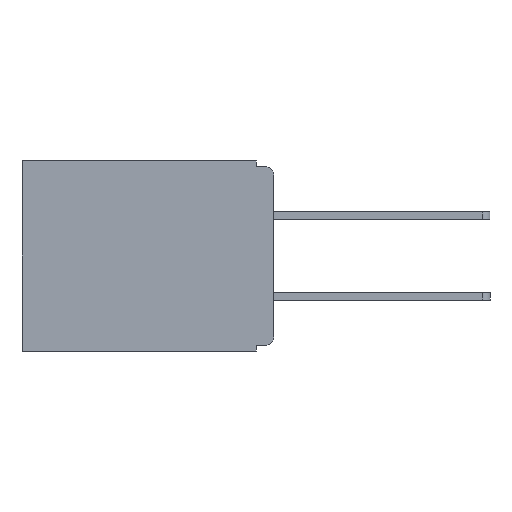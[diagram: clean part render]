
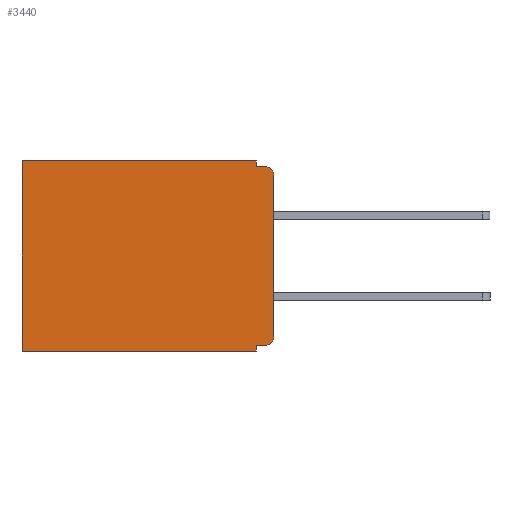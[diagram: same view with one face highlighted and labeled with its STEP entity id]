
A CAD part, left-side view. The second image highlights one B-rep face of the part: STEP entity #3440.
In plain terms, the highlighted planar face has unit normal (-1, 0, 0).
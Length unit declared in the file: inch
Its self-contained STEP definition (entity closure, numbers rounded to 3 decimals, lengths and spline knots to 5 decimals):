
#128 = EDGE_CURVE ( 'NONE', #9035, #3549, #1771, .T. ) ;
#164 = VERTEX_POINT ( 'NONE', #965 ) ;
#360 = EDGE_CURVE ( 'NONE', #1878, #3993, #12144, .T. ) ;
#444 = AXIS2_PLACEMENT_3D ( 'NONE', #8846, #1423, #1316 ) ;
#551 = LINE ( 'NONE', #1949, #5755 ) ;
#725 = AXIS2_PLACEMENT_3D ( 'NONE', #9932, #4043, #10915 ) ;
#837 = ORIENTED_EDGE ( 'NONE', *, *, #4532, .T. ) ;
#965 = CARTESIAN_POINT ( 'NONE',  ( 0.3, 0.437, -0.33 ) ) ;
#1316 = DIRECTION ( 'NONE',  ( 0., 0., -1. ) ) ;
#1423 = DIRECTION ( 'NONE',  ( 1., 0., 0. ) ) ;
#1461 = ORIENTED_EDGE ( 'NONE', *, *, #360, .F. ) ;
#1744 = CARTESIAN_POINT ( 'NONE',  ( 0.3, 0., -0.32 ) ) ;
#1756 = CARTESIAN_POINT ( 'NONE',  ( 0.3, 0.015, -0.305 ) ) ;
#1771 = LINE ( 'NONE', #1744, #4232 ) ;
#1878 = VERTEX_POINT ( 'NONE', #8219 ) ;
#1949 = CARTESIAN_POINT ( 'NONE',  ( 0.3, 0.031, -0.33 ) ) ;
#2025 = CARTESIAN_POINT ( 'NONE',  ( 0.3, 0.031, -0.33 ) ) ;
#2027 = FACE_OUTER_BOUND ( 'NONE', #11269, .T. ) ;
#2093 = CARTESIAN_POINT ( 'NONE',  ( 0.3, 0.015, -0.32 ) ) ;
#2695 = DIRECTION ( 'NONE',  ( 0., 0., -1. ) ) ;
#2806 = CARTESIAN_POINT ( 'NONE',  ( 0.3, 0., -0.01 ) ) ;
#2838 = DIRECTION ( 'NONE',  ( 0., 0., -1. ) ) ;
#3440 = ADVANCED_FACE ( 'NONE', ( #2027 ), #10654, .F. ) ;
#3549 = VERTEX_POINT ( 'NONE', #10870 ) ;
#3644 = CARTESIAN_POINT ( 'NONE',  ( 0.3, 0., -0.305 ) ) ;
#3832 = CARTESIAN_POINT ( 'NONE',  ( 0.3, 0.031, -0.01 ) ) ;
#3835 = VERTEX_POINT ( 'NONE', #5001 ) ;
#3843 = DIRECTION ( 'NONE',  ( 0., -1., 0. ) ) ;
#3993 = VERTEX_POINT ( 'NONE', #3644 ) ;
#4043 = DIRECTION ( 'NONE',  ( -1., 0., 0. ) ) ;
#4068 = VERTEX_POINT ( 'NONE', #6907 ) ;
#4093 = VECTOR ( 'NONE', #11956, 39.37008 ) ;
#4232 = VECTOR ( 'NONE', #11063, 39.37008 ) ;
#4323 = DIRECTION ( 'NONE',  ( 0., 0., -1. ) ) ;
#4532 = EDGE_CURVE ( 'NONE', #4068, #164, #7735, .T. ) ;
#4567 = ORIENTED_EDGE ( 'NONE', *, *, #12355, .F. ) ;
#4657 = LINE ( 'NONE', #8066, #7011 ) ;
#5001 = CARTESIAN_POINT ( 'NONE',  ( 0.3, 0.015, -0.01 ) ) ;
#5372 = ORIENTED_EDGE ( 'NONE', *, *, #6467, .F. ) ;
#5407 = ORIENTED_EDGE ( 'NONE', *, *, #10008, .F. ) ;
#5551 = LINE ( 'NONE', #12117, #7835 ) ;
#5755 = VECTOR ( 'NONE', #8007, 39.37008 ) ;
#5821 = CARTESIAN_POINT ( 'NONE',  ( 0.3, 0.031, 0. ) ) ;
#5886 = CARTESIAN_POINT ( 'NONE',  ( 0.3, 0.437, -0.33 ) ) ;
#6150 = CIRCLE ( 'NONE', #725, 0.015 ) ;
#6467 = EDGE_CURVE ( 'NONE', #12229, #3835, #8832, .T. ) ;
#6636 = EDGE_CURVE ( 'NONE', #8162, #4068, #4657, .T. ) ;
#6880 = VECTOR ( 'NONE', #3843, 39.37008 ) ;
#6907 = CARTESIAN_POINT ( 'NONE',  ( 0.3, 0.437, 0. ) ) ;
#6995 = EDGE_CURVE ( 'NONE', #9035, #3993, #10465, .T. ) ;
#7011 = VECTOR ( 'NONE', #12848, 39.37008 ) ;
#7239 = ORIENTED_EDGE ( 'NONE', *, *, #10126, .F. ) ;
#7428 = VECTOR ( 'NONE', #2695, 39.37008 ) ;
#7668 = VECTOR ( 'NONE', #11276, 39.37008 ) ;
#7735 = LINE ( 'NONE', #5886, #7428 ) ;
#7835 = VECTOR ( 'NONE', #4323, 39.37008 ) ;
#8007 = DIRECTION ( 'NONE',  ( 0., 0., -1. ) ) ;
#8066 = CARTESIAN_POINT ( 'NONE',  ( 0.3, 0., 0. ) ) ;
#8162 = VERTEX_POINT ( 'NONE', #5821 ) ;
#8219 = CARTESIAN_POINT ( 'NONE',  ( 0.3, 0., -0.025 ) ) ;
#8729 = ORIENTED_EDGE ( 'NONE', *, *, #10547, .T. ) ;
#8825 = DIRECTION ( 'NONE',  ( -1., 0., 0. ) ) ;
#8832 = LINE ( 'NONE', #2806, #6880 ) ;
#8846 = CARTESIAN_POINT ( 'NONE',  ( 0.3, 0., -0.33 ) ) ;
#8875 = CARTESIAN_POINT ( 'NONE',  ( 0.3, 0., -0.33 ) ) ;
#9035 = VERTEX_POINT ( 'NONE', #2093 ) ;
#9377 = ORIENTED_EDGE ( 'NONE', *, *, #128, .F. ) ;
#9932 = CARTESIAN_POINT ( 'NONE',  ( 0.3, 0.015, -0.025 ) ) ;
#10008 = EDGE_CURVE ( 'NONE', #11223, #164, #11881, .T. ) ;
#10026 = CARTESIAN_POINT ( 'NONE',  ( 0.3, 0., -0.33 ) ) ;
#10126 = EDGE_CURVE ( 'NONE', #8162, #12229, #5551, .T. ) ;
#10229 = ORIENTED_EDGE ( 'NONE', *, *, #6636, .T. ) ;
#10465 = CIRCLE ( 'NONE', #10719, 0.015 ) ;
#10547 = EDGE_CURVE ( 'NONE', #1878, #3835, #6150, .T. ) ;
#10654 = PLANE ( 'NONE',  #444 ) ;
#10719 = AXIS2_PLACEMENT_3D ( 'NONE', #1756, #8825, #2838 ) ;
#10870 = CARTESIAN_POINT ( 'NONE',  ( 0.3, 0.031, -0.32 ) ) ;
#10915 = DIRECTION ( 'NONE',  ( 0., 0., -1. ) ) ;
#11063 = DIRECTION ( 'NONE',  ( 0., 1., 0. ) ) ;
#11223 = VERTEX_POINT ( 'NONE', #2025 ) ;
#11269 = EDGE_LOOP ( 'NONE', ( #1461, #8729, #5372, #7239, #10229, #837, #5407, #4567, #9377, #12321 ) ) ;
#11276 = DIRECTION ( 'NONE',  ( 0., 0., -1. ) ) ;
#11881 = LINE ( 'NONE', #10026, #4093 ) ;
#11956 = DIRECTION ( 'NONE',  ( 0., 1., 0. ) ) ;
#12117 = CARTESIAN_POINT ( 'NONE',  ( 0.3, 0.031, 0. ) ) ;
#12144 = LINE ( 'NONE', #8875, #7668 ) ;
#12229 = VERTEX_POINT ( 'NONE', #3832 ) ;
#12321 = ORIENTED_EDGE ( 'NONE', *, *, #6995, .T. ) ;
#12355 = EDGE_CURVE ( 'NONE', #3549, #11223, #551, .T. ) ;
#12848 = DIRECTION ( 'NONE',  ( 0., 1., 0. ) ) ;
